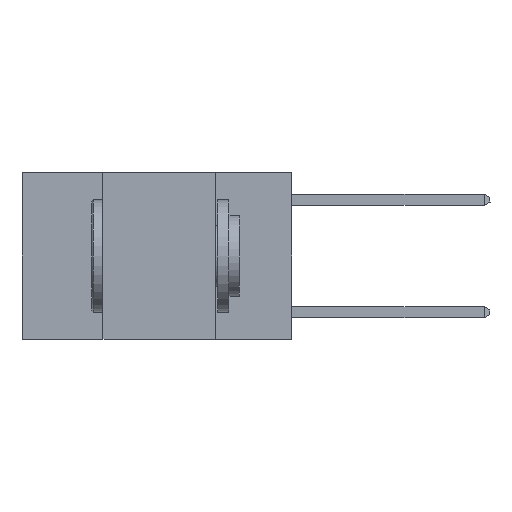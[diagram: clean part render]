
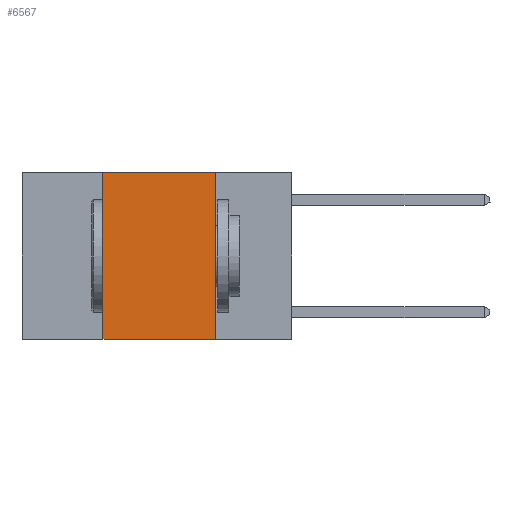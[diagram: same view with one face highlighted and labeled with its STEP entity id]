
A CAD part, left-side view. The second image highlights one B-rep face of the part: STEP entity #6567.
In plain terms, the highlighted planar face has unit normal (-1, 0, 0).
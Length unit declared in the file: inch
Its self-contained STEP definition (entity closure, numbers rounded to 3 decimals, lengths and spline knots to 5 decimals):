
#215 = CARTESIAN_POINT ( 'NONE',  ( 0., 0.42, 0. ) ) ;
#1967 = FACE_OUTER_BOUND ( 'NONE', #23503, .T. ) ;
#2166 = DIRECTION ( 'NONE',  ( 0., -1., 0. ) ) ;
#2752 = VERTEX_POINT ( 'NONE', #215 ) ;
#4191 = CARTESIAN_POINT ( 'NONE',  ( 0., 0.6, 0. ) ) ;
#4365 = ORIENTED_EDGE ( 'NONE', *, *, #8421, .F. ) ;
#5633 = EDGE_CURVE ( 'NONE', #2752, #25626, #25394, .T. ) ;
#5815 = CARTESIAN_POINT ( 'NONE',  ( 0., 0.6, 0. ) ) ;
#6567 = ADVANCED_FACE ( 'NONE', ( #1967 ), #8119, .F. ) ;
#7229 = DIRECTION ( 'NONE',  ( 0., 0., 1. ) ) ;
#8119 = PLANE ( 'NONE',  #29079 ) ;
#8421 = EDGE_CURVE ( 'NONE', #17941, #2752, #25905, .T. ) ;
#8686 = LINE ( 'NONE', #20198, #25840 ) ;
#10416 = DIRECTION ( 'NONE',  ( 0., 0., -1. ) ) ;
#11260 = VECTOR ( 'NONE', #26786, 39.37008 ) ;
#12701 = CARTESIAN_POINT ( 'NONE',  ( 0., 0.42, -0.37 ) ) ;
#13530 = DIRECTION ( 'NONE',  ( 0., 0., -1. ) ) ;
#14167 = EDGE_CURVE ( 'NONE', #25626, #27014, #8686, .T. ) ;
#14880 = CARTESIAN_POINT ( 'NONE',  ( 0., 0.17, 0. ) ) ;
#16163 = ORIENTED_EDGE ( 'NONE', *, *, #14167, .F. ) ;
#17291 = LINE ( 'NONE', #17940, #11260 ) ;
#17940 = CARTESIAN_POINT ( 'NONE',  ( 0., 0.6, -0.37 ) ) ;
#17941 = VERTEX_POINT ( 'NONE', #12701 ) ;
#18530 = CARTESIAN_POINT ( 'NONE',  ( 0., 0.42, 0. ) ) ;
#19525 = VECTOR ( 'NONE', #2166, 39.37008 ) ;
#19934 = ORIENTED_EDGE ( 'NONE', *, *, #5633, .F. ) ;
#20072 = VECTOR ( 'NONE', #7229, 39.37008 ) ;
#20198 = CARTESIAN_POINT ( 'NONE',  ( 0., 0.17, 0. ) ) ;
#23503 = EDGE_LOOP ( 'NONE', ( #16163, #19934, #4365, #26045 ) ) ;
#25394 = LINE ( 'NONE', #4191, #19525 ) ;
#25626 = VERTEX_POINT ( 'NONE', #14880 ) ;
#25840 = VECTOR ( 'NONE', #13530, 39.37008 ) ;
#25889 = EDGE_CURVE ( 'NONE', #17941, #27014, #17291, .T. ) ;
#25905 = LINE ( 'NONE', #18530, #20072 ) ;
#26045 = ORIENTED_EDGE ( 'NONE', *, *, #25889, .T. ) ;
#26338 = CARTESIAN_POINT ( 'NONE',  ( 0., 0.17, -0.37 ) ) ;
#26786 = DIRECTION ( 'NONE',  ( 0., -1., 0. ) ) ;
#27014 = VERTEX_POINT ( 'NONE', #26338 ) ;
#28176 = DIRECTION ( 'NONE',  ( 1., 0., 0. ) ) ;
#29079 = AXIS2_PLACEMENT_3D ( 'NONE', #5815, #28176, #10416 ) ;
